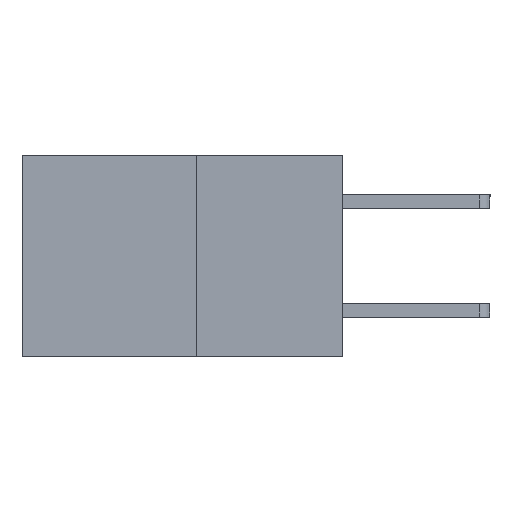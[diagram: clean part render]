
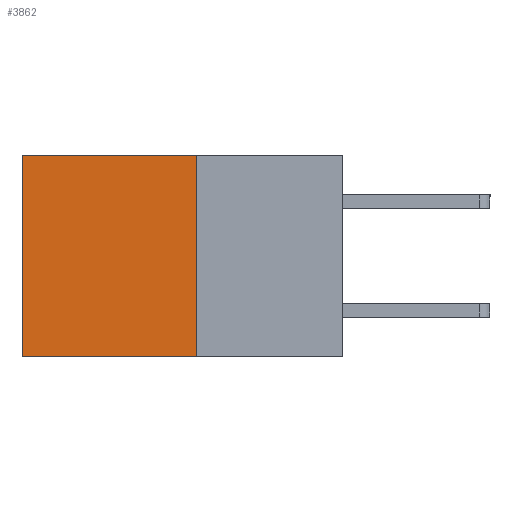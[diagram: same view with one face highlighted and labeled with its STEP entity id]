
A CAD part, left-side view. The second image highlights one B-rep face of the part: STEP entity #3862.
In plain terms, the highlighted planar face has unit normal (-1, 0, 0).
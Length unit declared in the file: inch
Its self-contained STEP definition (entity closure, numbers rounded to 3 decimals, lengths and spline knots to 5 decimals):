
#245 = EDGE_LOOP ( 'NONE', ( #4387, #3974, #3998, #1521 ) ) ;
#534 = VERTEX_POINT ( 'NONE', #1987 ) ;
#1297 = CARTESIAN_POINT ( 'NONE',  ( 0.277, 0.59, -0.37 ) ) ;
#1307 = VERTEX_POINT ( 'NONE', #10870 ) ;
#1521 = ORIENTED_EDGE ( 'NONE', *, *, #2228, .T. ) ;
#1586 = EDGE_CURVE ( 'NONE', #11920, #10731, #4293, .T. ) ;
#1694 = CARTESIAN_POINT ( 'NONE',  ( 0.277, 0.59, -0.37 ) ) ;
#1893 = EDGE_CURVE ( 'NONE', #534, #10731, #2179, .T. ) ;
#1987 = CARTESIAN_POINT ( 'NONE',  ( 0.277, 0.59, 0. ) ) ;
#2179 = LINE ( 'NONE', #1297, #4128 ) ;
#2194 = PLANE ( 'NONE',  #11449 ) ;
#2228 = EDGE_CURVE ( 'NONE', #1307, #534, #6059, .T. ) ;
#2253 = CARTESIAN_POINT ( 'NONE',  ( 0.277, 0.27, -0.37 ) ) ;
#2415 = DIRECTION ( 'NONE',  ( 0., 0., -1. ) ) ;
#2700 = DIRECTION ( 'NONE',  ( 0., 1., 0. ) ) ;
#3615 = VECTOR ( 'NONE', #7683, 39.37008 ) ;
#3862 = ADVANCED_FACE ( 'NONE', ( #6003 ), #2194, .F. ) ;
#3974 = ORIENTED_EDGE ( 'NONE', *, *, #1586, .F. ) ;
#3998 = ORIENTED_EDGE ( 'NONE', *, *, #7511, .F. ) ;
#4128 = VECTOR ( 'NONE', #2415, 39.37008 ) ;
#4293 = LINE ( 'NONE', #7176, #10991 ) ;
#4387 = ORIENTED_EDGE ( 'NONE', *, *, #1893, .T. ) ;
#5840 = CARTESIAN_POINT ( 'NONE',  ( 0.277, 0.27, -0.37 ) ) ;
#6003 = FACE_OUTER_BOUND ( 'NONE', #245, .T. ) ;
#6059 = LINE ( 'NONE', #7742, #3615 ) ;
#7176 = CARTESIAN_POINT ( 'NONE',  ( 0.277, 0.27, -0.37 ) ) ;
#7511 = EDGE_CURVE ( 'NONE', #1307, #11920, #9380, .T. ) ;
#7683 = DIRECTION ( 'NONE',  ( 0., 1., 0. ) ) ;
#7742 = CARTESIAN_POINT ( 'NONE',  ( 0.277, 0.27, 0. ) ) ;
#8324 = DIRECTION ( 'NONE',  ( 0., 0., -1. ) ) ;
#9127 = CARTESIAN_POINT ( 'NONE',  ( 0.277, 0.27, -0.37 ) ) ;
#9145 = VECTOR ( 'NONE', #8324, 39.37008 ) ;
#9380 = LINE ( 'NONE', #9127, #9145 ) ;
#9683 = DIRECTION ( 'NONE',  ( 0., 0., -1. ) ) ;
#9697 = DIRECTION ( 'NONE',  ( 1., 0., 0. ) ) ;
#10731 = VERTEX_POINT ( 'NONE', #1694 ) ;
#10870 = CARTESIAN_POINT ( 'NONE',  ( 0.277, 0.27, 0. ) ) ;
#10991 = VECTOR ( 'NONE', #2700, 39.37008 ) ;
#11449 = AXIS2_PLACEMENT_3D ( 'NONE', #2253, #9697, #9683 ) ;
#11920 = VERTEX_POINT ( 'NONE', #5840 ) ;
